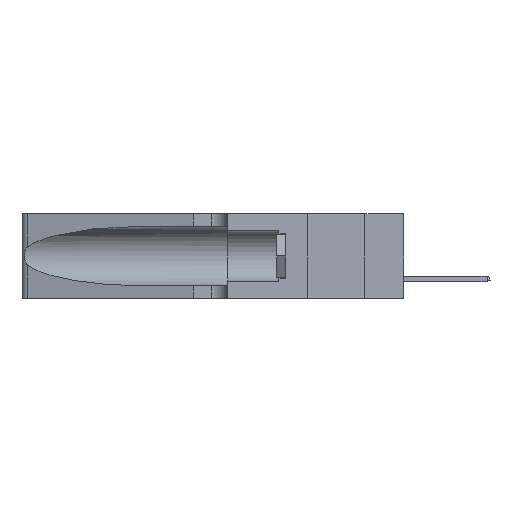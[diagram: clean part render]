
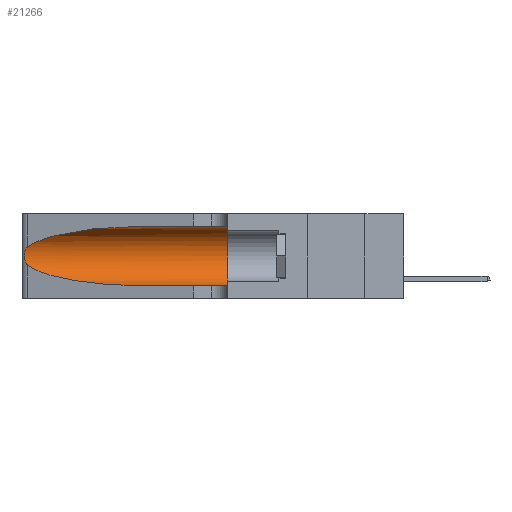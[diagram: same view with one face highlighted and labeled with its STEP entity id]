
A CAD part, left-side view. The second image highlights one B-rep face of the part: STEP entity #21266.
In plain terms, the highlighted cylindrical face has radius 3.308 mm (diameter 6.617 mm), a partial arc.
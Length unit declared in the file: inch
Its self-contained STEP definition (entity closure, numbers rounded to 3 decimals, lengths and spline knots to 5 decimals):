
#2576 = FACE_OUTER_BOUND ( 'NONE', #7539, .T. ) ;
#3379 = DIRECTION ( 'NONE',  ( 0., -1., 0. ) ) ;
#3552 = CARTESIAN_POINT ( 'NONE',  ( 0.25487, 1.22718, 0.22369 ) ) ;
#3720 = CARTESIAN_POINT ( 'NONE',  ( 0.25487, 1.22718, 0.14631 ) ) ;
#3786 = CYLINDRICAL_SURFACE ( 'NONE', #41127, 0.13025 ) ;
#4263 = ORIENTED_EDGE ( 'NONE', *, *, #15849, .T. ) ;
#4866 = DIRECTION ( 'NONE',  ( 0., 0., -1. ) ) ;
#7539 = EDGE_LOOP ( 'NONE', ( #48833, #4263, #13232, #8451, #41964, #33362 ) ) ;
#8451 = ORIENTED_EDGE ( 'NONE', *, *, #20436, .T. ) ;
#10114 = CARTESIAN_POINT ( 'NONE',  ( 0.1305, 0.72297, 0.05475 ) ) ;
#10878 = CARTESIAN_POINT ( 'NONE',  ( 0.25787, 1.23484, 0.2124 ) ) ;
#10911 = VERTEX_POINT ( 'NONE', #10987 ) ;
#10987 = CARTESIAN_POINT ( 'NONE',  ( 0.1305, 0.72297, 0.05475 ) ) ;
#12082 = CARTESIAN_POINT ( 'NONE',  ( 0.1305, 0.35, 0.31525 ) ) ;
#12547 = DIRECTION ( 'NONE',  ( 0., -1., 0. ) ) ;
#13232 = ORIENTED_EDGE ( 'NONE', *, *, #23404, .T. ) ;
#15512 = CARTESIAN_POINT ( 'NONE',  ( 0.25639, 1.23186, 0.15144 ) ) ;
#15849 = EDGE_CURVE ( 'NONE', #30023, #16300, #31499, .T. ) ;
#16280 = EDGE_CURVE ( 'NONE', #35262, #39131, #25752, .T. ) ;
#16300 = VERTEX_POINT ( 'NONE', #20287 ) ;
#17269 = CARTESIAN_POINT ( 'NONE',  ( 0.18966, 0.96281, 0.31525 ) ) ;
#18723 = CARTESIAN_POINT ( 'NONE',  ( 0.26018, 1.23835, 0.19895 ) ) ;
#18926 = CARTESIAN_POINT ( 'NONE',  ( 0.1305, 1.61858, 0.05475 ) ) ;
#19110 = CARTESIAN_POINT ( 'NONE',  ( 0.1305, 0.35, 0.185 ) ) ;
#19392 = CARTESIAN_POINT ( 'NONE',  ( 0.25789, 1.23486, 0.15765 ) ) ;
#20193 =( BOUNDED_CURVE ( )  B_SPLINE_CURVE ( 3, ( #45801, #29765, #30269, #10114 ),
 .UNSPECIFIED., .F., .T. ) 
 B_SPLINE_CURVE_WITH_KNOTS ( ( 4, 4 ),
 ( 3.44316, 4.71239 ),
 .UNSPECIFIED. ) 
 CURVE ( )  GEOMETRIC_REPRESENTATION_ITEM ( )  RATIONAL_B_SPLINE_CURVE ( ( 1., 0.87, 0.87, 1. ) ) 
 REPRESENTATION_ITEM ( '' )  );
#20287 = CARTESIAN_POINT ( 'NONE',  ( 0.25487, 1.22718, 0.14631 ) ) ;
#20436 = EDGE_CURVE ( 'NONE', #10911, #39131, #49670, .T. ) ;
#20537 = VERTEX_POINT ( 'NONE', #23854 ) ;
#21266 = ADVANCED_FACE ( 'NONE', ( #2576 ), #3786, .F. ) ;
#22975 = EDGE_CURVE ( 'NONE', #20537, #35262, #31437, .T. ) ;
#23150 = CARTESIAN_POINT ( 'NONE',  ( 0.26075, 1.23896, 0.178 ) ) ;
#23350 = CARTESIAN_POINT ( 'NONE',  ( 0.25555, 1.22993, 0.14849 ) ) ;
#23404 = EDGE_CURVE ( 'NONE', #16300, #10911, #20193, .T. ) ;
#23854 = CARTESIAN_POINT ( 'NONE',  ( 0.1305, 0.72297, 0.31525 ) ) ;
#24456 = CARTESIAN_POINT ( 'NONE',  ( 0.1305, 1.61858, 0.185 ) ) ;
#25752 = CIRCLE ( 'NONE', #49830, 0.13025 ) ;
#26484 = EDGE_CURVE ( 'NONE', #20537, #30023, #45898, .T. ) ;
#27067 = CARTESIAN_POINT ( 'NONE',  ( 0.25856, 1.23593, 0.16098 ) ) ;
#27484 = DIRECTION ( 'NONE',  ( 0., 0., 1. ) ) ;
#27533 = CARTESIAN_POINT ( 'NONE',  ( 0.25487, 1.22718, 0.22369 ) ) ;
#27743 = VECTOR ( 'NONE', #3379, 39.37008 ) ;
#29765 = CARTESIAN_POINT ( 'NONE',  ( 0.2373, 1.15595, 0.08982 ) ) ;
#30023 = VERTEX_POINT ( 'NONE', #27533 ) ;
#30269 = CARTESIAN_POINT ( 'NONE',  ( 0.18966, 0.96281, 0.05475 ) ) ;
#31437 = LINE ( 'NONE', #50312, #27743 ) ;
#31499 = B_SPLINE_CURVE_WITH_KNOTS ( 'NONE', 3,
 ( #3552, #42124, #46230, #10878, #46557, #18723, #42624, #23150, #50492, #27067, #19392, #15512, #23350, #3720 ),
 .UNSPECIFIED., .F., .F.,
 ( 4, 2, 2, 2, 2, 2, 4 ),
 ( 0., 0.00027, 0.00053, 0.00107, 0.0016, 0.00187, 0.00214 ),
 .UNSPECIFIED. ) ;
#33283 = CARTESIAN_POINT ( 'NONE',  ( 0.1305, 0.72297, 0.31525 ) ) ;
#33362 = ORIENTED_EDGE ( 'NONE', *, *, #22975, .F. ) ;
#34644 = CARTESIAN_POINT ( 'NONE',  ( 0.1305, 0.35, 0.05475 ) ) ;
#35014 = VECTOR ( 'NONE', #35154, 39.37008 ) ;
#35154 = DIRECTION ( 'NONE',  ( 0., -1., 0. ) ) ;
#35262 = VERTEX_POINT ( 'NONE', #12082 ) ;
#39131 = VERTEX_POINT ( 'NONE', #34644 ) ;
#41127 = AXIS2_PLACEMENT_3D ( 'NONE', #24456, #12547, #4866 ) ;
#41317 = CARTESIAN_POINT ( 'NONE',  ( 0.2373, 1.15595, 0.28018 ) ) ;
#41964 = ORIENTED_EDGE ( 'NONE', *, *, #16280, .F. ) ;
#42124 = CARTESIAN_POINT ( 'NONE',  ( 0.25555, 1.22994, 0.2215 ) ) ;
#42624 = CARTESIAN_POINT ( 'NONE',  ( 0.26075, 1.23896, 0.19203 ) ) ;
#43017 = DIRECTION ( 'NONE',  ( 0., 1., 0. ) ) ;
#44574 = CARTESIAN_POINT ( 'NONE',  ( 0.25487, 1.22718, 0.22369 ) ) ;
#45801 = CARTESIAN_POINT ( 'NONE',  ( 0.25487, 1.22718, 0.14631 ) ) ;
#45898 =( BOUNDED_CURVE ( )  B_SPLINE_CURVE ( 3, ( #33283, #17269, #41317, #44574 ),
 .UNSPECIFIED., .F., .F. ) 
 B_SPLINE_CURVE_WITH_KNOTS ( ( 4, 4 ),
 ( 1.5708, 2.84003 ),
 .UNSPECIFIED. ) 
 CURVE ( )  GEOMETRIC_REPRESENTATION_ITEM ( )  RATIONAL_B_SPLINE_CURVE ( ( 1., 0.87, 0.87, 1. ) ) 
 REPRESENTATION_ITEM ( '' )  );
#46230 = CARTESIAN_POINT ( 'NONE',  ( 0.25639, 1.23184, 0.21858 ) ) ;
#46557 = CARTESIAN_POINT ( 'NONE',  ( 0.25854, 1.2359, 0.20912 ) ) ;
#48833 = ORIENTED_EDGE ( 'NONE', *, *, #26484, .T. ) ;
#49670 = LINE ( 'NONE', #18926, #35014 ) ;
#49830 = AXIS2_PLACEMENT_3D ( 'NONE', #19110, #43017, #27484 ) ;
#50312 = CARTESIAN_POINT ( 'NONE',  ( 0.1305, 1.61858, 0.31525 ) ) ;
#50492 = CARTESIAN_POINT ( 'NONE',  ( 0.26017, 1.23833, 0.17102 ) ) ;
